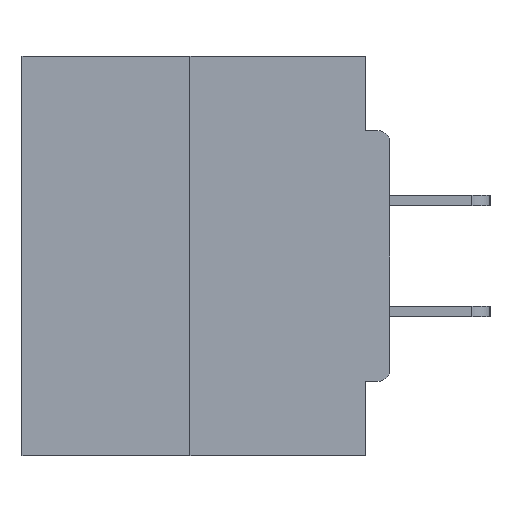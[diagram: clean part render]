
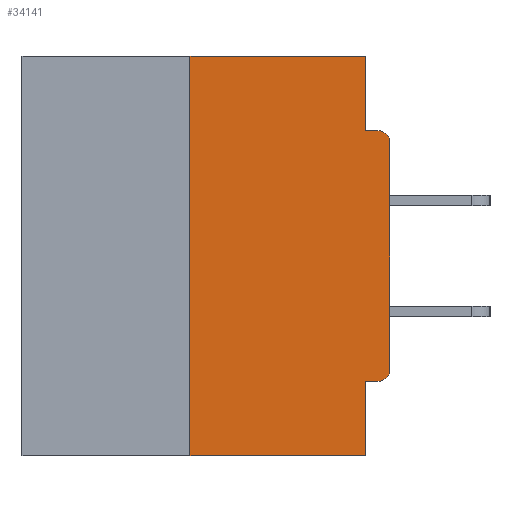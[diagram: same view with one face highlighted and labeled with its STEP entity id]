
A CAD part, left-side view. The second image highlights one B-rep face of the part: STEP entity #34141.
In plain terms, the highlighted planar face has unit normal (-1, 0, 0).
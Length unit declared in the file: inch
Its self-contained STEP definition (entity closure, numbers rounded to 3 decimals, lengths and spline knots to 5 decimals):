
#150 = VECTOR ( 'NONE', #18446, 39.37008 ) ;
#182 = LINE ( 'NONE', #24400, #1960 ) ;
#477 = ORIENTED_EDGE ( 'NONE', *, *, #19000, .T. ) ;
#1250 = DIRECTION ( 'NONE',  ( -1., 0., 0. ) ) ;
#1563 = CARTESIAN_POINT ( 'NONE',  ( 0., 0.031, 0. ) ) ;
#1960 = VECTOR ( 'NONE', #11172, 39.37008 ) ;
#2233 = CARTESIAN_POINT ( 'NONE',  ( 0., 0., 0. ) ) ;
#2453 = EDGE_CURVE ( 'NONE', #9164, #34785, #10395, .T. ) ;
#2682 = CARTESIAN_POINT ( 'NONE',  ( 0., 0.031, 0. ) ) ;
#3006 = CARTESIAN_POINT ( 'NONE',  ( 0., 0.25, 0. ) ) ;
#3072 = EDGE_LOOP ( 'NONE', ( #13636, #21672, #25658, #16152, #18568, #20503, #477, #31630, #9172, #3345 ) ) ;
#3345 = ORIENTED_EDGE ( 'NONE', *, *, #16034, .F. ) ;
#5068 = LINE ( 'NONE', #2233, #20104 ) ;
#5531 = CARTESIAN_POINT ( 'NONE',  ( 0., 0.031, -0.4065 ) ) ;
#6330 = VERTEX_POINT ( 'NONE', #26460 ) ;
#7318 = CARTESIAN_POINT ( 'NONE',  ( 0., 0., -0.4065 ) ) ;
#7503 = DIRECTION ( 'NONE',  ( -1., 0., 0. ) ) ;
#7537 = EDGE_CURVE ( 'NONE', #17509, #20154, #16917, .T. ) ;
#7542 = CIRCLE ( 'NONE', #8116, 0.015 ) ;
#8116 = AXIS2_PLACEMENT_3D ( 'NONE', #14762, #1250, #21917 ) ;
#8449 = VECTOR ( 'NONE', #18181, 39.37008 ) ;
#8736 = LINE ( 'NONE', #35158, #23437 ) ;
#8944 = VERTEX_POINT ( 'NONE', #14447 ) ;
#9026 = EDGE_CURVE ( 'NONE', #8944, #9164, #26384, .T. ) ;
#9071 = DIRECTION ( 'NONE',  ( 0., 0., 1. ) ) ;
#9164 = VERTEX_POINT ( 'NONE', #5531 ) ;
#9172 = ORIENTED_EDGE ( 'NONE', *, *, #31758, .F. ) ;
#10320 = AXIS2_PLACEMENT_3D ( 'NONE', #31757, #7503, #10338 ) ;
#10338 = DIRECTION ( 'NONE',  ( 0., 0., -1. ) ) ;
#10395 = LINE ( 'NONE', #10562, #12673 ) ;
#10406 = PLANE ( 'NONE',  #33157 ) ;
#10408 = LINE ( 'NONE', #15756, #150 ) ;
#10520 = VERTEX_POINT ( 'NONE', #2682 ) ;
#10557 = DIRECTION ( 'NONE',  ( 0., 0., 1. ) ) ;
#10562 = CARTESIAN_POINT ( 'NONE',  ( 0., 0.031, -0.5 ) ) ;
#10718 = DIRECTION ( 'NONE',  ( 0., -1., 0. ) ) ;
#11172 = DIRECTION ( 'NONE',  ( 0., -1., 0. ) ) ;
#11409 = VERTEX_POINT ( 'NONE', #20753 ) ;
#12103 = CARTESIAN_POINT ( 'NONE',  ( 0., 0.25, 0. ) ) ;
#12389 = LINE ( 'NONE', #1563, #13742 ) ;
#12673 = VECTOR ( 'NONE', #21254, 39.37008 ) ;
#13636 = ORIENTED_EDGE ( 'NONE', *, *, #30874, .F. ) ;
#13742 = VECTOR ( 'NONE', #15418, 39.37008 ) ;
#14447 = CARTESIAN_POINT ( 'NONE',  ( 0., 0.015, -0.4065 ) ) ;
#14762 = CARTESIAN_POINT ( 'NONE',  ( 0., 0.015, -0.3915 ) ) ;
#15086 = VERTEX_POINT ( 'NONE', #18226 ) ;
#15418 = DIRECTION ( 'NONE',  ( 0., 0., -1. ) ) ;
#15756 = CARTESIAN_POINT ( 'NONE',  ( 0., 0., -0.0935 ) ) ;
#16034 = EDGE_CURVE ( 'NONE', #10520, #31052, #12389, .T. ) ;
#16152 = ORIENTED_EDGE ( 'NONE', *, *, #2453, .F. ) ;
#16552 = CIRCLE ( 'NONE', #10320, 0.015 ) ;
#16917 = LINE ( 'NONE', #12103, #26059 ) ;
#17509 = VERTEX_POINT ( 'NONE', #27515 ) ;
#18181 = DIRECTION ( 'NONE',  ( 0., 1., 0. ) ) ;
#18226 = CARTESIAN_POINT ( 'NONE',  ( 0., 0.015, -0.0935 ) ) ;
#18446 = DIRECTION ( 'NONE',  ( 0., -1., 0. ) ) ;
#18568 = ORIENTED_EDGE ( 'NONE', *, *, #9026, .F. ) ;
#19000 = EDGE_CURVE ( 'NONE', #11409, #6330, #5068, .T. ) ;
#20104 = VECTOR ( 'NONE', #10557, 39.37008 ) ;
#20154 = VERTEX_POINT ( 'NONE', #3006 ) ;
#20503 = ORIENTED_EDGE ( 'NONE', *, *, #23536, .T. ) ;
#20753 = CARTESIAN_POINT ( 'NONE',  ( 0., 0., -0.3915 ) ) ;
#21254 = DIRECTION ( 'NONE',  ( 0., 0., -1. ) ) ;
#21267 = DIRECTION ( 'NONE',  ( 0., 0., -1. ) ) ;
#21672 = ORIENTED_EDGE ( 'NONE', *, *, #7537, .F. ) ;
#21917 = DIRECTION ( 'NONE',  ( 0., 0., -1. ) ) ;
#22808 = CARTESIAN_POINT ( 'NONE',  ( 0., 0.031, -0.0935 ) ) ;
#23437 = VECTOR ( 'NONE', #10718, 39.37008 ) ;
#23489 = CARTESIAN_POINT ( 'NONE',  ( 0., 0.031, -0.5 ) ) ;
#23536 = EDGE_CURVE ( 'NONE', #8944, #11409, #7542, .T. ) ;
#23960 = CARTESIAN_POINT ( 'NONE',  ( 0., 0.46, 0. ) ) ;
#24400 = CARTESIAN_POINT ( 'NONE',  ( 0., 0.46, -0.5 ) ) ;
#25658 = ORIENTED_EDGE ( 'NONE', *, *, #34474, .T. ) ;
#26059 = VECTOR ( 'NONE', #9071, 39.37008 ) ;
#26384 = LINE ( 'NONE', #7318, #8449 ) ;
#26403 = EDGE_CURVE ( 'NONE', #6330, #15086, #16552, .T. ) ;
#26460 = CARTESIAN_POINT ( 'NONE',  ( 0., 0., -0.1085 ) ) ;
#26981 = FACE_OUTER_BOUND ( 'NONE', #3072, .T. ) ;
#27515 = CARTESIAN_POINT ( 'NONE',  ( 0., 0.25, -0.5 ) ) ;
#30874 = EDGE_CURVE ( 'NONE', #20154, #10520, #8736, .T. ) ;
#31052 = VERTEX_POINT ( 'NONE', #22808 ) ;
#31630 = ORIENTED_EDGE ( 'NONE', *, *, #26403, .T. ) ;
#31757 = CARTESIAN_POINT ( 'NONE',  ( 0., 0.015, -0.1085 ) ) ;
#31758 = EDGE_CURVE ( 'NONE', #31052, #15086, #10408, .T. ) ;
#33157 = AXIS2_PLACEMENT_3D ( 'NONE', #23960, #34831, #21267 ) ;
#34141 = ADVANCED_FACE ( 'NONE', ( #26981 ), #10406, .F. ) ;
#34474 = EDGE_CURVE ( 'NONE', #17509, #34785, #182, .T. ) ;
#34785 = VERTEX_POINT ( 'NONE', #23489 ) ;
#34831 = DIRECTION ( 'NONE',  ( 1., 0., 0. ) ) ;
#35158 = CARTESIAN_POINT ( 'NONE',  ( 0., 0.46, 0. ) ) ;
